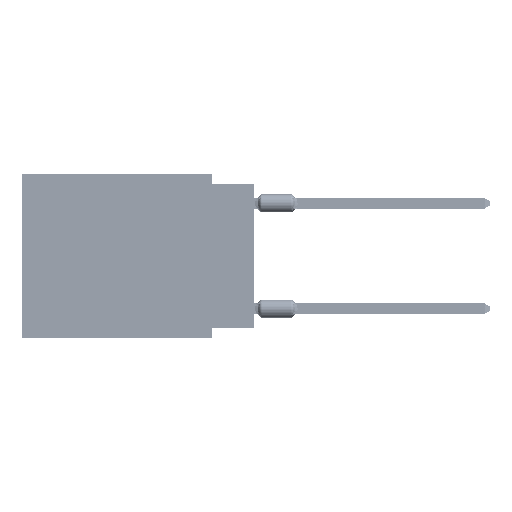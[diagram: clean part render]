
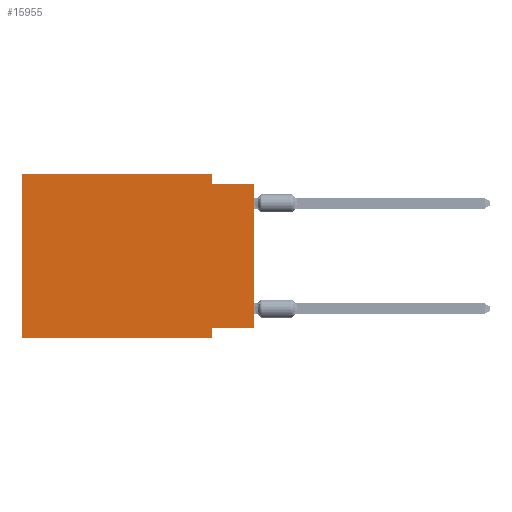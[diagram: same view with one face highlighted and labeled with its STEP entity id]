
A CAD part, left-side view. The second image highlights one B-rep face of the part: STEP entity #15955.
In plain terms, the highlighted planar face has unit normal (-1, 0, 0).
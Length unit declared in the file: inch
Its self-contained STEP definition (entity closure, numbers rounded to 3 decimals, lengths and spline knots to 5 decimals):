
#176 = VECTOR ( 'NONE', #65713, 39.37008 ) ;
#1106 = LINE ( 'NONE', #56739, #82011 ) ;
#1973 = DIRECTION ( 'NONE',  ( 0., 0., 1. ) ) ;
#3142 = VECTOR ( 'NONE', #1973, 39.37008 ) ;
#5175 = VERTEX_POINT ( 'NONE', #65178 ) ;
#5385 = DIRECTION ( 'NONE',  ( 0., 1., 0. ) ) ;
#6328 = EDGE_CURVE ( 'NONE', #24588, #29330, #84492, .T. ) ;
#6646 = CARTESIAN_POINT ( 'NONE',  ( 0., 0.55, -0.39 ) ) ;
#14874 = VERTEX_POINT ( 'NONE', #82982 ) ;
#15061 = DIRECTION ( 'NONE',  ( 0., 0., 1. ) ) ;
#15213 = EDGE_CURVE ( 'NONE', #67905, #14874, #63134, .T. ) ;
#15955 = ADVANCED_FACE ( 'NONE', ( #57601 ), #22160, .F. ) ;
#16853 = LINE ( 'NONE', #17726, #176 ) ;
#17726 = CARTESIAN_POINT ( 'NONE',  ( 0., 0., -0.025 ) ) ;
#20514 = VERTEX_POINT ( 'NONE', #62634 ) ;
#22160 = PLANE ( 'NONE',  #34180 ) ;
#22669 = CARTESIAN_POINT ( 'NONE',  ( 0., 0.55, 0. ) ) ;
#23024 = LINE ( 'NONE', #50402, #29686 ) ;
#24588 = VERTEX_POINT ( 'NONE', #31531 ) ;
#24905 = EDGE_CURVE ( 'NONE', #24588, #5175, #44892, .T. ) ;
#26917 = ORIENTED_EDGE ( 'NONE', *, *, #57556, .F. ) ;
#27639 = VECTOR ( 'NONE', #15061, 39.37008 ) ;
#29330 = VERTEX_POINT ( 'NONE', #75776 ) ;
#29686 = VECTOR ( 'NONE', #77732, 39.37008 ) ;
#31531 = CARTESIAN_POINT ( 'NONE',  ( 0., 0., -0.365 ) ) ;
#33236 = ORIENTED_EDGE ( 'NONE', *, *, #6328, .T. ) ;
#33906 = CARTESIAN_POINT ( 'NONE',  ( 0., 0.55, -0.39 ) ) ;
#34180 = AXIS2_PLACEMENT_3D ( 'NONE', #62987, #63878, #84944 ) ;
#34472 = DIRECTION ( 'NONE',  ( 0., -1., 0. ) ) ;
#36160 = ORIENTED_EDGE ( 'NONE', *, *, #58976, .F. ) ;
#42948 = VERTEX_POINT ( 'NONE', #54532 ) ;
#44892 = LINE ( 'NONE', #58792, #58087 ) ;
#46340 = ORIENTED_EDGE ( 'NONE', *, *, #76576, .F. ) ;
#47552 = EDGE_CURVE ( 'NONE', #61867, #42948, #23024, .T. ) ;
#49164 = CARTESIAN_POINT ( 'NONE',  ( 0., 0.55, 0. ) ) ;
#50402 = CARTESIAN_POINT ( 'NONE',  ( 0., 0.55, 0. ) ) ;
#51294 = VECTOR ( 'NONE', #34472, 39.37008 ) ;
#52391 = CARTESIAN_POINT ( 'NONE',  ( 0., 0.1, 0. ) ) ;
#53277 = LINE ( 'NONE', #52391, #59149 ) ;
#54532 = CARTESIAN_POINT ( 'NONE',  ( 0., 0.1, 0. ) ) ;
#55859 = DIRECTION ( 'NONE',  ( 0., 0., -1. ) ) ;
#56739 = CARTESIAN_POINT ( 'NONE',  ( 0., 0.1, -0.39 ) ) ;
#57151 = CARTESIAN_POINT ( 'NONE',  ( 0., 0., 0. ) ) ;
#57556 = EDGE_CURVE ( 'NONE', #67905, #61867, #76935, .T. ) ;
#57601 = FACE_OUTER_BOUND ( 'NONE', #77723, .T. ) ;
#58087 = VECTOR ( 'NONE', #5385, 39.37008 ) ;
#58792 = CARTESIAN_POINT ( 'NONE',  ( 0., 0., -0.365 ) ) ;
#58976 = EDGE_CURVE ( 'NONE', #42948, #20514, #53277, .T. ) ;
#59149 = VECTOR ( 'NONE', #66713, 39.37008 ) ;
#61867 = VERTEX_POINT ( 'NONE', #22669 ) ;
#62634 = CARTESIAN_POINT ( 'NONE',  ( 0., 0.1, -0.025 ) ) ;
#62987 = CARTESIAN_POINT ( 'NONE',  ( 0., 0.55, 0. ) ) ;
#63134 = LINE ( 'NONE', #6646, #51294 ) ;
#63878 = DIRECTION ( 'NONE',  ( 1., 0., 0. ) ) ;
#65116 = ORIENTED_EDGE ( 'NONE', *, *, #15213, .T. ) ;
#65178 = CARTESIAN_POINT ( 'NONE',  ( 0., 0.1, -0.365 ) ) ;
#65713 = DIRECTION ( 'NONE',  ( 0., -1., 0. ) ) ;
#66713 = DIRECTION ( 'NONE',  ( 0., 0., -1. ) ) ;
#67905 = VERTEX_POINT ( 'NONE', #33906 ) ;
#70022 = ORIENTED_EDGE ( 'NONE', *, *, #73598, .F. ) ;
#73598 = EDGE_CURVE ( 'NONE', #20514, #29330, #16853, .T. ) ;
#75776 = CARTESIAN_POINT ( 'NONE',  ( 0., 0., -0.025 ) ) ;
#76576 = EDGE_CURVE ( 'NONE', #5175, #14874, #1106, .T. ) ;
#76935 = LINE ( 'NONE', #49164, #27639 ) ;
#77723 = EDGE_LOOP ( 'NONE', ( #33236, #70022, #36160, #88332, #26917, #65116, #46340, #81382 ) ) ;
#77732 = DIRECTION ( 'NONE',  ( 0., -1., 0. ) ) ;
#81382 = ORIENTED_EDGE ( 'NONE', *, *, #24905, .F. ) ;
#82011 = VECTOR ( 'NONE', #55859, 39.37008 ) ;
#82982 = CARTESIAN_POINT ( 'NONE',  ( 0., 0.1, -0.39 ) ) ;
#84492 = LINE ( 'NONE', #57151, #3142 ) ;
#84944 = DIRECTION ( 'NONE',  ( 0., 0., -1. ) ) ;
#88332 = ORIENTED_EDGE ( 'NONE', *, *, #47552, .F. ) ;
